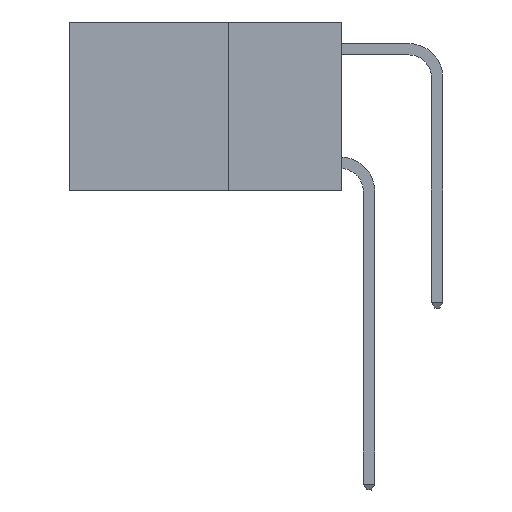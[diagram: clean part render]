
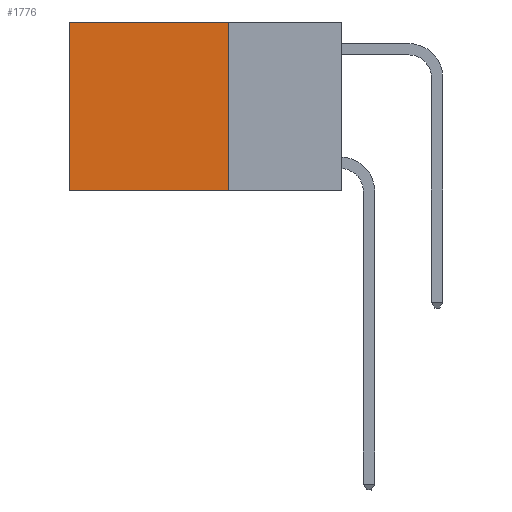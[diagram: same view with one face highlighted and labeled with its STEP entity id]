
A CAD part, left-side view. The second image highlights one B-rep face of the part: STEP entity #1776.
In plain terms, the highlighted planar face has unit normal (-1, 0, 0).
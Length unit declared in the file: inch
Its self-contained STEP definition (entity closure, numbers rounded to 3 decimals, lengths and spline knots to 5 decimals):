
#149 = DIRECTION ( 'NONE',  ( 1., 0., 0. ) ) ;
#622 = VERTEX_POINT ( 'NONE', #12023 ) ;
#630 = CARTESIAN_POINT ( 'NONE',  ( 0.2625, 0.25, -0.37 ) ) ;
#943 = LINE ( 'NONE', #7686, #10644 ) ;
#1776 = ADVANCED_FACE ( 'NONE', ( #5542 ), #6168, .F. ) ;
#2274 = LINE ( 'NONE', #4897, #6963 ) ;
#2397 = EDGE_CURVE ( 'NONE', #7878, #8658, #2274, .T. ) ;
#3609 = EDGE_LOOP ( 'NONE', ( #5062, #5739, #7048, #10959 ) ) ;
#3800 = DIRECTION ( 'NONE',  ( 0., 0., -1. ) ) ;
#4897 = CARTESIAN_POINT ( 'NONE',  ( 0.2625, 0.6, 0. ) ) ;
#5062 = ORIENTED_EDGE ( 'NONE', *, *, #2397, .T. ) ;
#5542 = FACE_OUTER_BOUND ( 'NONE', #3609, .T. ) ;
#5727 = LINE ( 'NONE', #11199, #10338 ) ;
#5739 = ORIENTED_EDGE ( 'NONE', *, *, #10204, .F. ) ;
#6168 = PLANE ( 'NONE',  #9309 ) ;
#6555 = VERTEX_POINT ( 'NONE', #7588 ) ;
#6829 = CARTESIAN_POINT ( 'NONE',  ( 0.2625, 0.6, 0. ) ) ;
#6963 = VECTOR ( 'NONE', #3800, 39.37008 ) ;
#7048 = ORIENTED_EDGE ( 'NONE', *, *, #8422, .F. ) ;
#7112 = CARTESIAN_POINT ( 'NONE',  ( 0.2625, 0.6, -0.37 ) ) ;
#7282 = VECTOR ( 'NONE', #9129, 39.37008 ) ;
#7588 = CARTESIAN_POINT ( 'NONE',  ( 0.2625, 0.25, 0. ) ) ;
#7686 = CARTESIAN_POINT ( 'NONE',  ( 0.2625, 0.25, 0. ) ) ;
#7878 = VERTEX_POINT ( 'NONE', #6829 ) ;
#8052 = DIRECTION ( 'NONE',  ( 0., 0., -1. ) ) ;
#8173 = CARTESIAN_POINT ( 'NONE',  ( 0.2625, 0.25, 0. ) ) ;
#8422 = EDGE_CURVE ( 'NONE', #6555, #622, #943, .T. ) ;
#8658 = VERTEX_POINT ( 'NONE', #7112 ) ;
#8849 = EDGE_CURVE ( 'NONE', #6555, #7878, #5727, .T. ) ;
#9129 = DIRECTION ( 'NONE',  ( 0., 1., 0. ) ) ;
#9309 = AXIS2_PLACEMENT_3D ( 'NONE', #8173, #149, #8052 ) ;
#9531 = DIRECTION ( 'NONE',  ( 0., 0., -1. ) ) ;
#9728 = LINE ( 'NONE', #630, #7282 ) ;
#10204 = EDGE_CURVE ( 'NONE', #622, #8658, #9728, .T. ) ;
#10270 = DIRECTION ( 'NONE',  ( 0., 1., 0. ) ) ;
#10338 = VECTOR ( 'NONE', #10270, 39.37008 ) ;
#10644 = VECTOR ( 'NONE', #9531, 39.37008 ) ;
#10959 = ORIENTED_EDGE ( 'NONE', *, *, #8849, .T. ) ;
#11199 = CARTESIAN_POINT ( 'NONE',  ( 0.2625, 0.25, 0. ) ) ;
#12023 = CARTESIAN_POINT ( 'NONE',  ( 0.2625, 0.25, -0.37 ) ) ;
